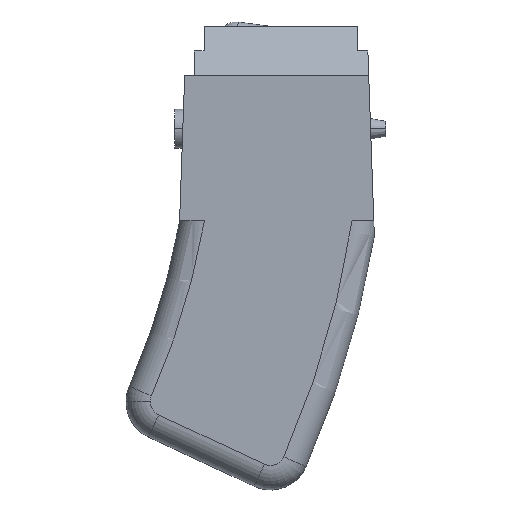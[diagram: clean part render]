
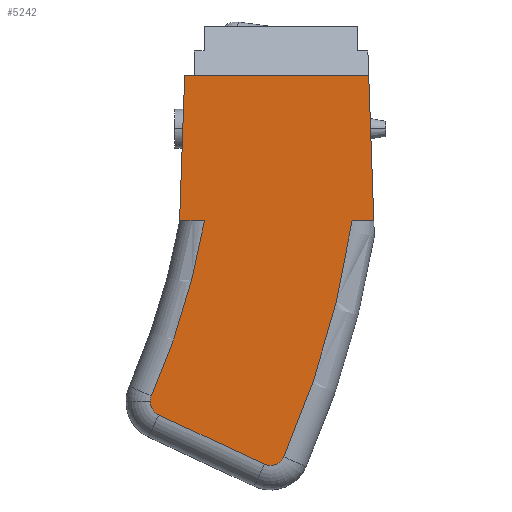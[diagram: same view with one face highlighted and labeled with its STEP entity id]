
A CAD part, top view. The second image highlights one B-rep face of the part: STEP entity #5242.
In plain terms, the highlighted planar face has unit normal (0, 0, 1).
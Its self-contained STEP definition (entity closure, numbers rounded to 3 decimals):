
#94 = DIRECTION ( 'NONE',  ( 0., 0., 1. ) ) ;
#214 = VERTEX_POINT ( 'NONE', #7807 ) ;
#319 = CARTESIAN_POINT ( 'NONE',  ( -17.469, -28., 16. ) ) ;
#560 = VECTOR ( 'NONE', #3541, 1000. ) ;
#578 = ORIENTED_EDGE ( 'NONE', *, *, #4516, .T. ) ;
#676 = CIRCLE ( 'NONE', #3606, 3. ) ;
#779 = EDGE_CURVE ( 'NONE', #4271, #5379, #7485, .T. ) ;
#850 = CARTESIAN_POINT ( 'NONE',  ( -21.556, 2., 16. ) ) ;
#963 = VERTEX_POINT ( 'NONE', #1951 ) ;
#974 = AXIS2_PLACEMENT_3D ( 'NONE', #4433, #94, #5154 ) ;
#1003 = CARTESIAN_POINT ( 'NONE',  ( 17.397, -28., 16. ) ) ;
#1123 = CARTESIAN_POINT ( 'NONE',  ( -28.626, -65.241, 16. ) ) ;
#1173 = AXIS2_PLACEMENT_3D ( 'NONE', #5660, #1307, #6389 ) ;
#1307 = DIRECTION ( 'NONE',  ( 0., 0., 1. ) ) ;
#1536 = ORIENTED_EDGE ( 'NONE', *, *, #8691, .T. ) ;
#1568 = CIRCLE ( 'NONE', #7915, 160. ) ;
#1676 = VERTEX_POINT ( 'NONE', #2048 ) ;
#1744 = ORIENTED_EDGE ( 'NONE', *, *, #9329, .T. ) ;
#1951 = CARTESIAN_POINT ( 'NONE',  ( -5.137, -78.105, 16. ) ) ;
#2048 = CARTESIAN_POINT ( 'NONE',  ( -1.123, -76.596, 16. ) ) ;
#2081 = DIRECTION ( 'NONE',  ( 0., 0., 1. ) ) ;
#2097 = CARTESIAN_POINT ( 'NONE',  ( -25.626, -65.241, 16. ) ) ;
#2255 = LINE ( 'NONE', #7864, #560 ) ;
#2348 = EDGE_CURVE ( 'NONE', #4271, #214, #2255, .T. ) ;
#2427 = VERTEX_POINT ( 'NONE', #3127 ) ;
#2505 = DIRECTION ( 'NONE',  ( 0., 0., -1. ) ) ;
#2645 = CARTESIAN_POINT ( 'NONE',  ( -15.974, -73.052, 16. ) ) ;
#2654 = CARTESIAN_POINT ( 'NONE',  ( 17.397, -28., 16. ) ) ;
#2827 = DIRECTION ( 'NONE',  ( 1., 0., 0. ) ) ;
#2933 = DIRECTION ( 'NONE',  ( 0., 0., 1. ) ) ;
#3127 = CARTESIAN_POINT ( 'NONE',  ( -28.375, -64.04, 16. ) ) ;
#3138 = DIRECTION ( 'NONE',  ( -1., 0., 0. ) ) ;
#3221 = VECTOR ( 'NONE', #8894, 1000. ) ;
#3352 = VECTOR ( 'NONE', #8695, 1000. ) ;
#3407 = EDGE_CURVE ( 'NONE', #7367, #963, #6655, .T. ) ;
#3443 = CARTESIAN_POINT ( 'NONE',  ( 17.397, 2., 16. ) ) ;
#3541 = DIRECTION ( 'NONE',  ( -0.035, 0.999, 0. ) ) ;
#3589 = ORIENTED_EDGE ( 'NONE', *, *, #5318, .T. ) ;
#3606 = AXIS2_PLACEMENT_3D ( 'NONE', #2097, #7176, #2827 ) ;
#3993 = VECTOR ( 'NONE', #5634, 1000. ) ;
#4023 = ORIENTED_EDGE ( 'NONE', *, *, #4638, .T. ) ;
#4035 = EDGE_CURVE ( 'NONE', #7663, #4131, #5270, .T. ) ;
#4091 = ORIENTED_EDGE ( 'NONE', *, *, #4035, .F. ) ;
#4106 = DIRECTION ( 'NONE',  ( 0.906, -0.423, 0. ) ) ;
#4131 = VERTEX_POINT ( 'NONE', #5195 ) ;
#4209 = CARTESIAN_POINT ( 'NONE',  ( -16.396, -73.958, 16. ) ) ;
#4244 = EDGE_CURVE ( 'NONE', #4131, #6732, #7102, .T. ) ;
#4246 = LINE ( 'NONE', #3443, #3993 ) ;
#4271 = VERTEX_POINT ( 'NONE', #1003 ) ;
#4433 = CARTESIAN_POINT ( 'NONE',  ( -175., 0., 16. ) ) ;
#4470 = EDGE_CURVE ( 'NONE', #963, #1676, #4752, .T. ) ;
#4516 = EDGE_CURVE ( 'NONE', #5080, #7367, #676, .T. ) ;
#4580 = CARTESIAN_POINT ( 'NONE',  ( -21.508, 3.359, 16. ) ) ;
#4638 = EDGE_CURVE ( 'NONE', #1676, #5379, #7259, .T. ) ;
#4715 = VECTOR ( 'NONE', #4106, 1000. ) ;
#4752 = CIRCLE ( 'NONE', #1173, 3. ) ;
#4808 = EDGE_LOOP ( 'NONE', ( #4023, #7776, #7691, #1536, #6382, #4091, #3589, #1744, #578, #9363, #6967 ) ) ;
#5024 = CIRCLE ( 'NONE', #7581, 3. ) ;
#5080 = VERTEX_POINT ( 'NONE', #1123 ) ;
#5154 = DIRECTION ( 'NONE',  ( 1., 0., 0. ) ) ;
#5195 = CARTESIAN_POINT ( 'NONE',  ( -22.603, -28., 16. ) ) ;
#5242 = ADVANCED_FACE ( 'NONE', ( #7564 ), #6397, .T. ) ;
#5270 = LINE ( 'NONE', #2654, #3352 ) ;
#5318 = EDGE_CURVE ( 'NONE', #7663, #2427, #1568, .T. ) ;
#5345 = VECTOR ( 'NONE', #3138, 1000. ) ;
#5379 = VERTEX_POINT ( 'NONE', #7631 ) ;
#5634 = DIRECTION ( 'NONE',  ( -1., 0., 0. ) ) ;
#5660 = CARTESIAN_POINT ( 'NONE',  ( -3.869, -75.386, 16. ) ) ;
#6382 = ORIENTED_EDGE ( 'NONE', *, *, #4244, .F. ) ;
#6389 = DIRECTION ( 'NONE',  ( 1., 0., 0. ) ) ;
#6397 = PLANE ( 'NONE',  #6951 ) ;
#6655 = LINE ( 'NONE', #2645, #4715 ) ;
#6732 = VERTEX_POINT ( 'NONE', #850 ) ;
#6845 = CARTESIAN_POINT ( 'NONE',  ( -175., 0., 16. ) ) ;
#6951 = AXIS2_PLACEMENT_3D ( 'NONE', #4209, #2081, #7156 ) ;
#6967 = ORIENTED_EDGE ( 'NONE', *, *, #4470, .T. ) ;
#7102 = LINE ( 'NONE', #4580, #3221 ) ;
#7156 = DIRECTION ( 'NONE',  ( 1., 0., 0. ) ) ;
#7176 = DIRECTION ( 'NONE',  ( 0., 0., 1. ) ) ;
#7259 = CIRCLE ( 'NONE', #974, 190. ) ;
#7276 = CARTESIAN_POINT ( 'NONE',  ( -25.626, -65.241, 16. ) ) ;
#7367 = VERTEX_POINT ( 'NONE', #9308 ) ;
#7474 = CARTESIAN_POINT ( 'NONE',  ( 17.397, -28., 16. ) ) ;
#7485 = LINE ( 'NONE', #7474, #5345 ) ;
#7564 = FACE_OUTER_BOUND ( 'NONE', #4808, .T. ) ;
#7574 = DIRECTION ( 'NONE',  ( 1., 0., 0. ) ) ;
#7581 = AXIS2_PLACEMENT_3D ( 'NONE', #7276, #2933, #7985 ) ;
#7631 = CARTESIAN_POINT ( 'NONE',  ( 12.926, -28., 16. ) ) ;
#7663 = VERTEX_POINT ( 'NONE', #319 ) ;
#7691 = ORIENTED_EDGE ( 'NONE', *, *, #2348, .T. ) ;
#7776 = ORIENTED_EDGE ( 'NONE', *, *, #779, .F. ) ;
#7807 = CARTESIAN_POINT ( 'NONE',  ( 16.349, 2., 16. ) ) ;
#7864 = CARTESIAN_POINT ( 'NONE',  ( 16.35, 1.963, 16. ) ) ;
#7915 = AXIS2_PLACEMENT_3D ( 'NONE', #6845, #2505, #7574 ) ;
#7985 = DIRECTION ( 'NONE',  ( 1., 0., 0. ) ) ;
#8691 = EDGE_CURVE ( 'NONE', #214, #6732, #4246, .T. ) ;
#8695 = DIRECTION ( 'NONE',  ( -1., 0., 0. ) ) ;
#8894 = DIRECTION ( 'NONE',  ( 0.035, 0.999, 0. ) ) ;
#9308 = CARTESIAN_POINT ( 'NONE',  ( -26.894, -67.96, 16. ) ) ;
#9329 = EDGE_CURVE ( 'NONE', #2427, #5080, #5024, .T. ) ;
#9363 = ORIENTED_EDGE ( 'NONE', *, *, #3407, .T. ) ;
